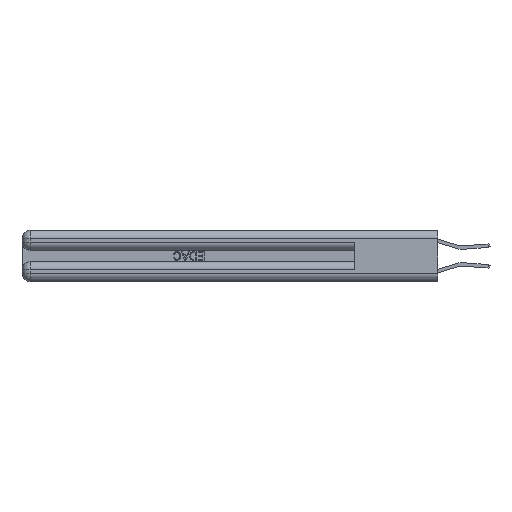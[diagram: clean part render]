
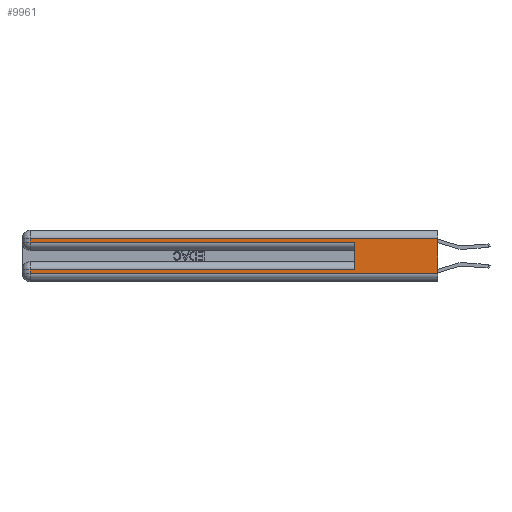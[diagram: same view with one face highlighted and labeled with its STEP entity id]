
A CAD part, left-side view. The second image highlights one B-rep face of the part: STEP entity #9961.
In plain terms, the highlighted planar face has unit normal (-1, 0, 0).
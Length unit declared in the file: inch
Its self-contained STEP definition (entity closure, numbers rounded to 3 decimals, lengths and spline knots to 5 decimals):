
#759 = ORIENTED_EDGE ( 'NONE', *, *, #11670, .T. ) ;
#1130 = LINE ( 'NONE', #21828, #2073 ) ;
#1670 = EDGE_CURVE ( 'NONE', #25931, #17838, #1130, .T. ) ;
#2073 = VECTOR ( 'NONE', #3575, 39.37008 ) ;
#2372 = EDGE_LOOP ( 'NONE', ( #18068, #3269, #24228, #20864, #8732, #25899, #759, #4504 ) ) ;
#2388 = DIRECTION ( 'NONE',  ( 0., 0., -1. ) ) ;
#3038 = CARTESIAN_POINT ( 'NONE',  ( 0., 0., 0.285 ) ) ;
#3217 = VERTEX_POINT ( 'NONE', #19193 ) ;
#3269 = ORIENTED_EDGE ( 'NONE', *, *, #4699, .T. ) ;
#3575 = DIRECTION ( 'NONE',  ( 0., 0., 1. ) ) ;
#3753 = VERTEX_POINT ( 'NONE', #8056 ) ;
#4145 = CARTESIAN_POINT ( 'NONE',  ( 0., 0.6, 0.285 ) ) ;
#4504 = ORIENTED_EDGE ( 'NONE', *, *, #5119, .T. ) ;
#4592 = DIRECTION ( 'NONE',  ( 0., 1., 0. ) ) ;
#4699 = EDGE_CURVE ( 'NONE', #23469, #3217, #11426, .T. ) ;
#5119 = EDGE_CURVE ( 'NONE', #26526, #3753, #17769, .T. ) ;
#5535 = CARTESIAN_POINT ( 'NONE',  ( 0., 0., 0.37 ) ) ;
#5771 = DIRECTION ( 'NONE',  ( 0., -1., 0. ) ) ;
#6095 = CARTESIAN_POINT ( 'NONE',  ( 0., 2.94, 0.085 ) ) ;
#8056 = CARTESIAN_POINT ( 'NONE',  ( 0., 0., 0.06 ) ) ;
#8411 = PLANE ( 'NONE',  #16644 ) ;
#8646 = EDGE_CURVE ( 'NONE', #3217, #20587, #29342, .T. ) ;
#8732 = ORIENTED_EDGE ( 'NONE', *, *, #1670, .F. ) ;
#9961 = ADVANCED_FACE ( 'NONE', ( #17825 ), #8411, .F. ) ;
#10160 = CARTESIAN_POINT ( 'NONE',  ( 0., 0., 0.31 ) ) ;
#10674 = EDGE_CURVE ( 'NONE', #20587, #17838, #14594, .T. ) ;
#11003 = DIRECTION ( 'NONE',  ( 1., 0., 0. ) ) ;
#11086 = DIRECTION ( 'NONE',  ( 0., -1., 0. ) ) ;
#11411 = CARTESIAN_POINT ( 'NONE',  ( 0., 2.94, 0.285 ) ) ;
#11426 = LINE ( 'NONE', #17797, #14225 ) ;
#11670 = EDGE_CURVE ( 'NONE', #27963, #26526, #18655, .T. ) ;
#12685 = DIRECTION ( 'NONE',  ( 0., 0., -1. ) ) ;
#13725 = VECTOR ( 'NONE', #2388, 39.37008 ) ;
#14225 = VECTOR ( 'NONE', #4592, 39.37008 ) ;
#14594 = LINE ( 'NONE', #3038, #16224 ) ;
#16224 = VECTOR ( 'NONE', #5771, 39.37008 ) ;
#16518 = CARTESIAN_POINT ( 'NONE',  ( 0., 2.94, 0.37 ) ) ;
#16644 = AXIS2_PLACEMENT_3D ( 'NONE', #20241, #11003, #20544 ) ;
#17769 = LINE ( 'NONE', #24603, #28312 ) ;
#17797 = CARTESIAN_POINT ( 'NONE',  ( 0., 0., 0.31 ) ) ;
#17825 = FACE_OUTER_BOUND ( 'NONE', #2372, .T. ) ;
#17838 = VERTEX_POINT ( 'NONE', #4145 ) ;
#18068 = ORIENTED_EDGE ( 'NONE', *, *, #27503, .F. ) ;
#18655 = LINE ( 'NONE', #16518, #13725 ) ;
#18946 = CARTESIAN_POINT ( 'NONE',  ( 0., 0., 0.085 ) ) ;
#19193 = CARTESIAN_POINT ( 'NONE',  ( 0., 2.94, 0.31 ) ) ;
#19964 = VECTOR ( 'NONE', #23532, 39.37008 ) ;
#20234 = CARTESIAN_POINT ( 'NONE',  ( 0., 2.94, 0.37 ) ) ;
#20241 = CARTESIAN_POINT ( 'NONE',  ( 0., 0., 0.37 ) ) ;
#20544 = DIRECTION ( 'NONE',  ( 0., 0., -1. ) ) ;
#20587 = VERTEX_POINT ( 'NONE', #11411 ) ;
#20864 = ORIENTED_EDGE ( 'NONE', *, *, #10674, .T. ) ;
#20876 = VECTOR ( 'NONE', #29486, 39.37008 ) ;
#21828 = CARTESIAN_POINT ( 'NONE',  ( 0., 0.6, 0.145 ) ) ;
#23469 = VERTEX_POINT ( 'NONE', #10160 ) ;
#23532 = DIRECTION ( 'NONE',  ( 0., 1., 0. ) ) ;
#23738 = CARTESIAN_POINT ( 'NONE',  ( 0., 2.94, 0.06 ) ) ;
#24123 = LINE ( 'NONE', #18946, #19964 ) ;
#24228 = ORIENTED_EDGE ( 'NONE', *, *, #8646, .T. ) ;
#24603 = CARTESIAN_POINT ( 'NONE',  ( 0., 0., 0.06 ) ) ;
#25899 = ORIENTED_EDGE ( 'NONE', *, *, #29109, .T. ) ;
#25931 = VERTEX_POINT ( 'NONE', #27118 ) ;
#26526 = VERTEX_POINT ( 'NONE', #23738 ) ;
#27118 = CARTESIAN_POINT ( 'NONE',  ( 0., 0.6, 0.085 ) ) ;
#27297 = VECTOR ( 'NONE', #12685, 39.37008 ) ;
#27503 = EDGE_CURVE ( 'NONE', #23469, #3753, #28605, .T. ) ;
#27963 = VERTEX_POINT ( 'NONE', #6095 ) ;
#28312 = VECTOR ( 'NONE', #11086, 39.37008 ) ;
#28605 = LINE ( 'NONE', #5535, #27297 ) ;
#29109 = EDGE_CURVE ( 'NONE', #25931, #27963, #24123, .T. ) ;
#29342 = LINE ( 'NONE', #20234, #20876 ) ;
#29486 = DIRECTION ( 'NONE',  ( 0., 0., -1. ) ) ;
